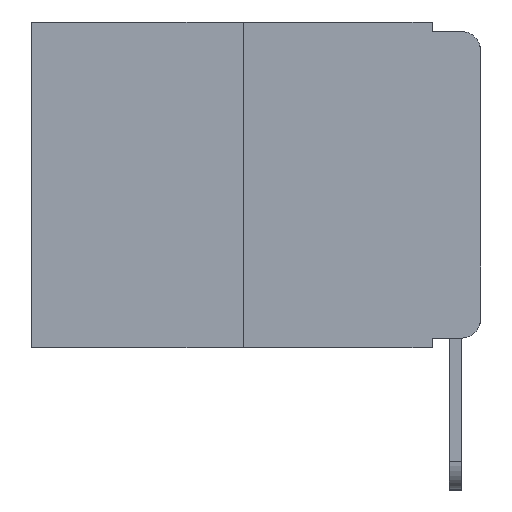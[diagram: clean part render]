
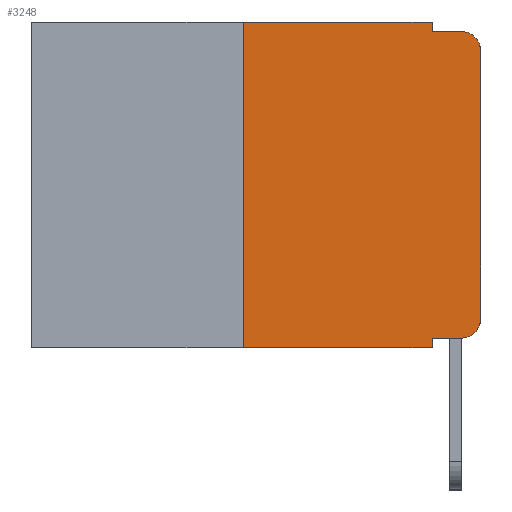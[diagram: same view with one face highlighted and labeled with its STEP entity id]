
A CAD part, left-side view. The second image highlights one B-rep face of the part: STEP entity #3248.
In plain terms, the highlighted planar face has unit normal (-1, 0, 0).
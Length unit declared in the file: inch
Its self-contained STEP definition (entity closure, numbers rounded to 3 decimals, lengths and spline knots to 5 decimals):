
#19 = VERTEX_POINT ( 'NONE', #3627 ) ;
#455 = ORIENTED_EDGE ( 'NONE', *, *, #4737, .F. ) ;
#766 = CARTESIAN_POINT ( 'NONE',  ( 0., 0.051, -0.01 ) ) ;
#1100 = DIRECTION ( 'NONE',  ( 0., 0., -1. ) ) ;
#1213 = LINE ( 'NONE', #14329, #4183 ) ;
#1314 = ORIENTED_EDGE ( 'NONE', *, *, #13463, .T. ) ;
#1508 = CARTESIAN_POINT ( 'NONE',  ( 0., 0.051, 0. ) ) ;
#1680 = LINE ( 'NONE', #8249, #7014 ) ;
#2007 = DIRECTION ( 'NONE',  ( -1., 0., 0. ) ) ;
#2306 = EDGE_CURVE ( 'NONE', #6831, #6277, #8857, .T. ) ;
#2399 = AXIS2_PLACEMENT_3D ( 'NONE', #8751, #2007, #11598 ) ;
#2493 = ORIENTED_EDGE ( 'NONE', *, *, #3994, .T. ) ;
#3019 = ORIENTED_EDGE ( 'NONE', *, *, #15961, .F. ) ;
#3176 = CARTESIAN_POINT ( 'NONE',  ( 0., 0., -0.03 ) ) ;
#3197 = DIRECTION ( 'NONE',  ( 0., -1., 0. ) ) ;
#3248 = ADVANCED_FACE ( 'NONE', ( #7958 ), #7845, .F. ) ;
#3627 = CARTESIAN_POINT ( 'NONE',  ( 0., 0.051, -0.343 ) ) ;
#3864 = DIRECTION ( 'NONE',  ( 0., -1., 0. ) ) ;
#3994 = EDGE_CURVE ( 'NONE', #17013, #8171, #16995, .T. ) ;
#4183 = VECTOR ( 'NONE', #8883, 39.37008 ) ;
#4648 = LINE ( 'NONE', #6124, #9341 ) ;
#4737 = EDGE_CURVE ( 'NONE', #11022, #5561, #4648, .T. ) ;
#5432 = ORIENTED_EDGE ( 'NONE', *, *, #16617, .T. ) ;
#5561 = VERTEX_POINT ( 'NONE', #1508 ) ;
#6124 = CARTESIAN_POINT ( 'NONE',  ( 0., 0.473, 0. ) ) ;
#6151 = VERTEX_POINT ( 'NONE', #766 ) ;
#6218 = DIRECTION ( 'NONE',  ( 0., 0., 1. ) ) ;
#6270 = CARTESIAN_POINT ( 'NONE',  ( 0., 0., -0.313 ) ) ;
#6277 = VERTEX_POINT ( 'NONE', #3176 ) ;
#6350 = VECTOR ( 'NONE', #6218, 39.37008 ) ;
#6413 = CARTESIAN_POINT ( 'NONE',  ( 0., 0.02, -0.313 ) ) ;
#6516 = VECTOR ( 'NONE', #12574, 39.37008 ) ;
#6575 = CIRCLE ( 'NONE', #9682, 0.02 ) ;
#6825 = ORIENTED_EDGE ( 'NONE', *, *, #2306, .T. ) ;
#6831 = VERTEX_POINT ( 'NONE', #6270 ) ;
#7014 = VECTOR ( 'NONE', #9730, 39.37008 ) ;
#7034 = VECTOR ( 'NONE', #13197, 39.37008 ) ;
#7101 = EDGE_LOOP ( 'NONE', ( #6825, #5432, #8156, #12741, #455, #8884, #1314, #3019, #2493, #11587 ) ) ;
#7785 = DIRECTION ( 'NONE',  ( -1., 0., 0. ) ) ;
#7845 = PLANE ( 'NONE',  #17168 ) ;
#7958 = FACE_OUTER_BOUND ( 'NONE', #7101, .T. ) ;
#8156 = ORIENTED_EDGE ( 'NONE', *, *, #9584, .F. ) ;
#8171 = VERTEX_POINT ( 'NONE', #9759 ) ;
#8249 = CARTESIAN_POINT ( 'NONE',  ( 0., 0.051, 0. ) ) ;
#8749 = CARTESIAN_POINT ( 'NONE',  ( 0., 0.473, -0.343 ) ) ;
#8751 = CARTESIAN_POINT ( 'NONE',  ( 0., 0.02, -0.03 ) ) ;
#8857 = LINE ( 'NONE', #14111, #6516 ) ;
#8883 = DIRECTION ( 'NONE',  ( 0., 0., -1. ) ) ;
#8884 = ORIENTED_EDGE ( 'NONE', *, *, #12960, .F. ) ;
#8904 = CARTESIAN_POINT ( 'NONE',  ( 0., 0.25, 0. ) ) ;
#8915 = LINE ( 'NONE', #8904, #6350 ) ;
#9195 = VERTEX_POINT ( 'NONE', #15021 ) ;
#9238 = CARTESIAN_POINT ( 'NONE',  ( 0., 0.02, -0.01 ) ) ;
#9341 = VECTOR ( 'NONE', #14441, 39.37008 ) ;
#9584 = EDGE_CURVE ( 'NONE', #6151, #14507, #13453, .T. ) ;
#9621 = CARTESIAN_POINT ( 'NONE',  ( 0., 0.051, -0.333 ) ) ;
#9682 = AXIS2_PLACEMENT_3D ( 'NONE', #6413, #7785, #17267 ) ;
#9730 = DIRECTION ( 'NONE',  ( 0., 0., -1. ) ) ;
#9759 = CARTESIAN_POINT ( 'NONE',  ( 0., 0.02, -0.333 ) ) ;
#9869 = VECTOR ( 'NONE', #3864, 39.37008 ) ;
#10653 = CARTESIAN_POINT ( 'NONE',  ( 0., 0.051, -0.01 ) ) ;
#11022 = VERTEX_POINT ( 'NONE', #16499 ) ;
#11423 = CIRCLE ( 'NONE', #2399, 0.02 ) ;
#11587 = ORIENTED_EDGE ( 'NONE', *, *, #12459, .T. ) ;
#11598 = DIRECTION ( 'NONE',  ( 0., 0., -1. ) ) ;
#11725 = CARTESIAN_POINT ( 'NONE',  ( 0., 0.051, -0.333 ) ) ;
#12459 = EDGE_CURVE ( 'NONE', #8171, #6831, #6575, .T. ) ;
#12574 = DIRECTION ( 'NONE',  ( 0., 0., 1. ) ) ;
#12741 = ORIENTED_EDGE ( 'NONE', *, *, #15614, .F. ) ;
#12960 = EDGE_CURVE ( 'NONE', #9195, #11022, #8915, .T. ) ;
#13197 = DIRECTION ( 'NONE',  ( 0., -1., 0. ) ) ;
#13453 = LINE ( 'NONE', #10653, #9869 ) ;
#13463 = EDGE_CURVE ( 'NONE', #9195, #19, #14386, .T. ) ;
#14111 = CARTESIAN_POINT ( 'NONE',  ( 0., 0., 0. ) ) ;
#14329 = CARTESIAN_POINT ( 'NONE',  ( 0., 0.051, 0. ) ) ;
#14386 = LINE ( 'NONE', #8749, #16111 ) ;
#14441 = DIRECTION ( 'NONE',  ( 0., -1., 0. ) ) ;
#14507 = VERTEX_POINT ( 'NONE', #9238 ) ;
#14675 = CARTESIAN_POINT ( 'NONE',  ( 0., 0.473, 0. ) ) ;
#15021 = CARTESIAN_POINT ( 'NONE',  ( 0., 0.25, -0.343 ) ) ;
#15614 = EDGE_CURVE ( 'NONE', #5561, #6151, #1680, .T. ) ;
#15961 = EDGE_CURVE ( 'NONE', #17013, #19, #1213, .T. ) ;
#16111 = VECTOR ( 'NONE', #3197, 39.37008 ) ;
#16499 = CARTESIAN_POINT ( 'NONE',  ( 0., 0.25, 0. ) ) ;
#16617 = EDGE_CURVE ( 'NONE', #6277, #14507, #11423, .T. ) ;
#16995 = LINE ( 'NONE', #11725, #7034 ) ;
#17013 = VERTEX_POINT ( 'NONE', #9621 ) ;
#17168 = AXIS2_PLACEMENT_3D ( 'NONE', #14675, #17322, #1100 ) ;
#17267 = DIRECTION ( 'NONE',  ( 0., 0., -1. ) ) ;
#17322 = DIRECTION ( 'NONE',  ( 1., 0., 0. ) ) ;
